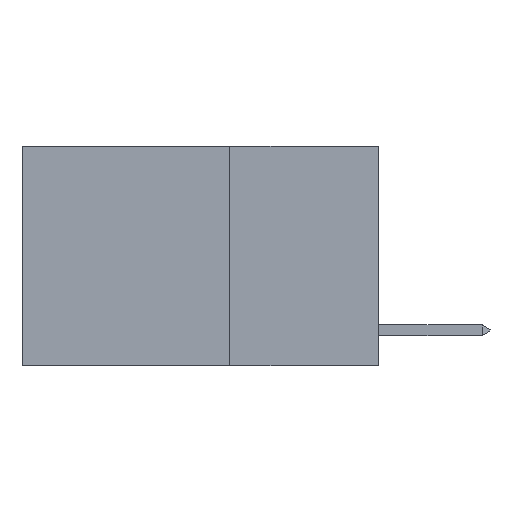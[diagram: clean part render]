
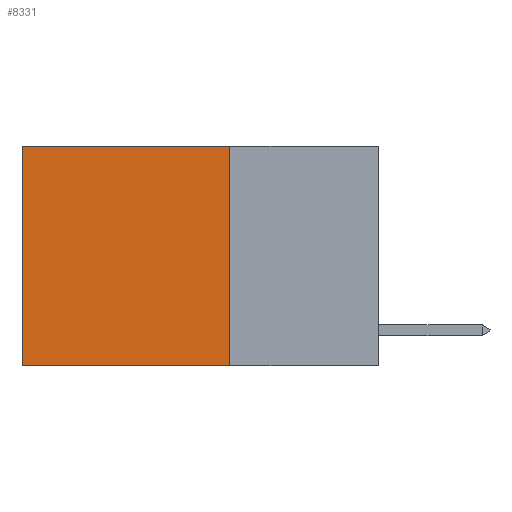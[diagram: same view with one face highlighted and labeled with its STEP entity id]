
A CAD part, left-side view. The second image highlights one B-rep face of the part: STEP entity #8331.
In plain terms, the highlighted planar face has unit normal (-1, 0, 0).
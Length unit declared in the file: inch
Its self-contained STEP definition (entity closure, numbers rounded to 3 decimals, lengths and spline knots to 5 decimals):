
#1258 = EDGE_CURVE ( 'NONE', #5346, #4244, #6750, .T. ) ;
#1274 = ORIENTED_EDGE ( 'NONE', *, *, #9158, .T. ) ;
#1739 = AXIS2_PLACEMENT_3D ( 'NONE', #2680, #6481, #9585 ) ;
#2654 = ORIENTED_EDGE ( 'NONE', *, *, #1258, .T. ) ;
#2680 = CARTESIAN_POINT ( 'NONE',  ( 0.2625, 0.25, 0. ) ) ;
#2681 = VECTOR ( 'NONE', #11946, 39.37008 ) ;
#2685 = ORIENTED_EDGE ( 'NONE', *, *, #11626, .F. ) ;
#3148 = DIRECTION ( 'NONE',  ( 0., 0., -1. ) ) ;
#3204 = EDGE_CURVE ( 'NONE', #11685, #3747, #5336, .T. ) ;
#3747 = VERTEX_POINT ( 'NONE', #11654 ) ;
#4127 = VECTOR ( 'NONE', #8377, 39.37008 ) ;
#4244 = VERTEX_POINT ( 'NONE', #6949 ) ;
#4435 = EDGE_LOOP ( 'NONE', ( #1274, #6827, #2685, #2654 ) ) ;
#4686 = LINE ( 'NONE', #7081, #5307 ) ;
#4985 = VECTOR ( 'NONE', #7155, 39.37008 ) ;
#5307 = VECTOR ( 'NONE', #3148, 39.37008 ) ;
#5336 = LINE ( 'NONE', #7008, #2681 ) ;
#5346 = VERTEX_POINT ( 'NONE', #12653 ) ;
#5457 = FACE_OUTER_BOUND ( 'NONE', #4435, .T. ) ;
#5522 = CARTESIAN_POINT ( 'NONE',  ( 0.2625, 0.25, 0. ) ) ;
#6481 = DIRECTION ( 'NONE',  ( 1., 0., 0. ) ) ;
#6653 = LINE ( 'NONE', #8151, #4985 ) ;
#6750 = LINE ( 'NONE', #5522, #4127 ) ;
#6827 = ORIENTED_EDGE ( 'NONE', *, *, #3204, .F. ) ;
#6949 = CARTESIAN_POINT ( 'NONE',  ( 0.2625, 0.6, 0. ) ) ;
#7008 = CARTESIAN_POINT ( 'NONE',  ( 0.2625, 0.25, -0.37 ) ) ;
#7081 = CARTESIAN_POINT ( 'NONE',  ( 0.2625, 0.25, 0. ) ) ;
#7155 = DIRECTION ( 'NONE',  ( 0., 0., -1. ) ) ;
#8151 = CARTESIAN_POINT ( 'NONE',  ( 0.2625, 0.6, 0. ) ) ;
#8331 = ADVANCED_FACE ( 'NONE', ( #5457 ), #8635, .F. ) ;
#8377 = DIRECTION ( 'NONE',  ( 0., 1., 0. ) ) ;
#8635 = PLANE ( 'NONE',  #1739 ) ;
#9107 = CARTESIAN_POINT ( 'NONE',  ( 0.2625, 0.25, -0.37 ) ) ;
#9158 = EDGE_CURVE ( 'NONE', #4244, #3747, #6653, .T. ) ;
#9585 = DIRECTION ( 'NONE',  ( 0., 0., -1. ) ) ;
#11626 = EDGE_CURVE ( 'NONE', #5346, #11685, #4686, .T. ) ;
#11654 = CARTESIAN_POINT ( 'NONE',  ( 0.2625, 0.6, -0.37 ) ) ;
#11685 = VERTEX_POINT ( 'NONE', #9107 ) ;
#11946 = DIRECTION ( 'NONE',  ( 0., 1., 0. ) ) ;
#12653 = CARTESIAN_POINT ( 'NONE',  ( 0.2625, 0.25, 0. ) ) ;
